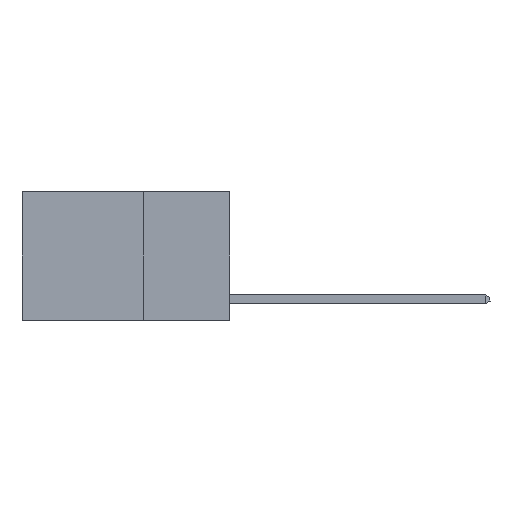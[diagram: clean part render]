
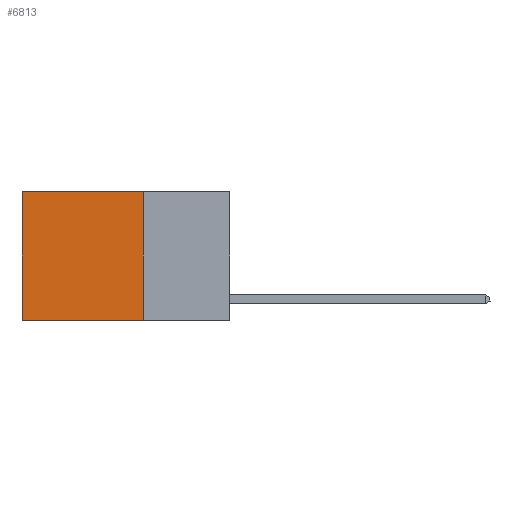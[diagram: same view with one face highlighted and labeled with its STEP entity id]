
A CAD part, left-side view. The second image highlights one B-rep face of the part: STEP entity #6813.
In plain terms, the highlighted planar face has unit normal (-1, 0, 0).
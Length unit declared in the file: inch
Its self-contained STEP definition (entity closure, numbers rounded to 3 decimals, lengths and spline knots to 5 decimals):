
#197 = VECTOR ( 'NONE', #1959, 39.37008 ) ;
#761 = FACE_OUTER_BOUND ( 'NONE', #3716, .T. ) ;
#1828 = CARTESIAN_POINT ( 'NONE',  ( 0.2625, 0.25, 0. ) ) ;
#1959 = DIRECTION ( 'NONE',  ( 0., 0., -1. ) ) ;
#2280 = EDGE_CURVE ( 'NONE', #16525, #16031, #11259, .T. ) ;
#3716 = EDGE_LOOP ( 'NONE', ( #15069, #19237, #22485, #16080 ) ) ;
#3750 = CARTESIAN_POINT ( 'NONE',  ( 0.2625, 0.25, 0. ) ) ;
#4403 = LINE ( 'NONE', #11854, #24579 ) ;
#4533 = LINE ( 'NONE', #17651, #4856 ) ;
#4856 = VECTOR ( 'NONE', #13235, 39.37008 ) ;
#6120 = DIRECTION ( 'NONE',  ( 1., 0., 0. ) ) ;
#6216 = DIRECTION ( 'NONE',  ( 0., 0., -1. ) ) ;
#6732 = EDGE_CURVE ( 'NONE', #16655, #16031, #4403, .T. ) ;
#6813 = ADVANCED_FACE ( 'NONE', ( #761 ), #20536, .F. ) ;
#8105 = CARTESIAN_POINT ( 'NONE',  ( 0.2625, 0.25, 0. ) ) ;
#9222 = CARTESIAN_POINT ( 'NONE',  ( 0.2625, 0.6, -0.37 ) ) ;
#10850 = EDGE_CURVE ( 'NONE', #20857, #16525, #14084, .T. ) ;
#11259 = LINE ( 'NONE', #24755, #197 ) ;
#11641 = CARTESIAN_POINT ( 'NONE',  ( 0.2625, 0.25, -0.37 ) ) ;
#11854 = CARTESIAN_POINT ( 'NONE',  ( 0.2625, 0.25, -0.37 ) ) ;
#13235 = DIRECTION ( 'NONE',  ( 0., 0., -1. ) ) ;
#14084 = LINE ( 'NONE', #3750, #14408 ) ;
#14169 = AXIS2_PLACEMENT_3D ( 'NONE', #1828, #6120, #6216 ) ;
#14205 = DIRECTION ( 'NONE',  ( 0., 1., 0. ) ) ;
#14408 = VECTOR ( 'NONE', #14205, 39.37008 ) ;
#15069 = ORIENTED_EDGE ( 'NONE', *, *, #2280, .T. ) ;
#16031 = VERTEX_POINT ( 'NONE', #9222 ) ;
#16080 = ORIENTED_EDGE ( 'NONE', *, *, #10850, .T. ) ;
#16525 = VERTEX_POINT ( 'NONE', #19637 ) ;
#16655 = VERTEX_POINT ( 'NONE', #11641 ) ;
#17651 = CARTESIAN_POINT ( 'NONE',  ( 0.2625, 0.25, 0. ) ) ;
#19237 = ORIENTED_EDGE ( 'NONE', *, *, #6732, .F. ) ;
#19637 = CARTESIAN_POINT ( 'NONE',  ( 0.2625, 0.6, 0. ) ) ;
#20099 = DIRECTION ( 'NONE',  ( 0., 1., 0. ) ) ;
#20536 = PLANE ( 'NONE',  #14169 ) ;
#20857 = VERTEX_POINT ( 'NONE', #8105 ) ;
#22485 = ORIENTED_EDGE ( 'NONE', *, *, #23294, .F. ) ;
#23294 = EDGE_CURVE ( 'NONE', #20857, #16655, #4533, .T. ) ;
#24579 = VECTOR ( 'NONE', #20099, 39.37008 ) ;
#24755 = CARTESIAN_POINT ( 'NONE',  ( 0.2625, 0.6, 0. ) ) ;
